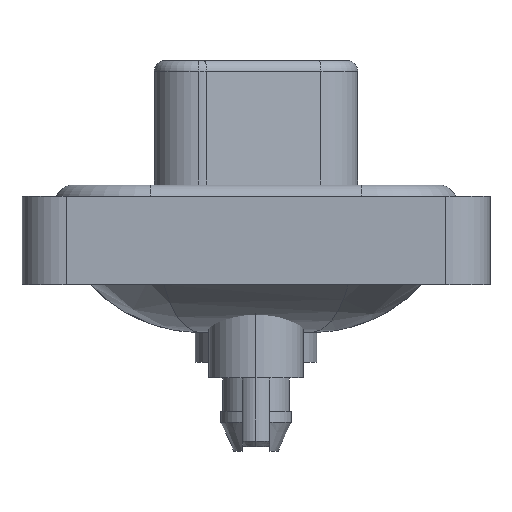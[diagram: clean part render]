
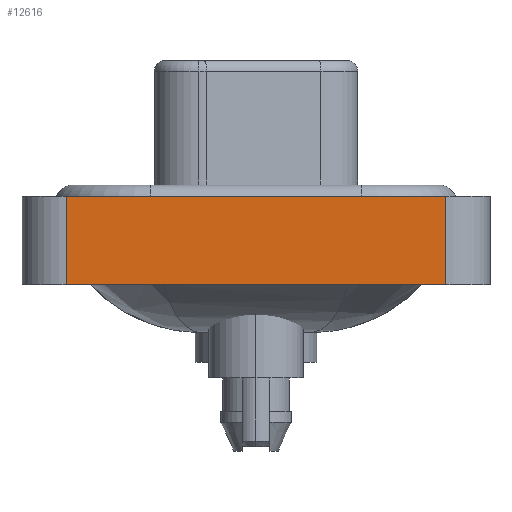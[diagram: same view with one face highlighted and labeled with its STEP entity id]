
A CAD part, left-side view. The second image highlights one B-rep face of the part: STEP entity #12616.
In plain terms, the highlighted planar face has unit normal (-1, 0, 0).
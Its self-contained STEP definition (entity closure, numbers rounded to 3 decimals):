
#95 = CARTESIAN_POINT ( 'NONE',  ( -7.25, 8.55, -3.6 ) ) ;
#122 = EDGE_CURVE ( 'NONE', #6247, #7674, #1466, .T. ) ;
#132 = LINE ( 'NONE', #12544, #2816 ) ;
#764 = CARTESIAN_POINT ( 'NONE',  ( -7.25, -8.55, 0.4 ) ) ;
#1466 = LINE ( 'NONE', #95, #2359 ) ;
#2124 = CARTESIAN_POINT ( 'NONE',  ( -7.25, 8.55, -3.6 ) ) ;
#2359 = VECTOR ( 'NONE', #2757, 1000. ) ;
#2703 = VECTOR ( 'NONE', #5706, 1000. ) ;
#2757 = DIRECTION ( 'NONE',  ( 0., 0., 1. ) ) ;
#2816 = VECTOR ( 'NONE', #13908, 1000. ) ;
#3711 = LINE ( 'NONE', #7516, #14394 ) ;
#4063 = CARTESIAN_POINT ( 'NONE',  ( -7.25, 8.55, 0.4 ) ) ;
#4376 = ORIENTED_EDGE ( 'NONE', *, *, #5754, .F. ) ;
#4644 = VERTEX_POINT ( 'NONE', #13628 ) ;
#5287 = ORIENTED_EDGE ( 'NONE', *, *, #11710, .T. ) ;
#5706 = DIRECTION ( 'NONE',  ( 0., -1., 0. ) ) ;
#5754 = EDGE_CURVE ( 'NONE', #7674, #15015, #9117, .T. ) ;
#5914 = AXIS2_PLACEMENT_3D ( 'NONE', #7771, #11454, #10336 ) ;
#6247 = VERTEX_POINT ( 'NONE', #2124 ) ;
#7322 = CARTESIAN_POINT ( 'NONE',  ( -7.25, -8.55, 0.4 ) ) ;
#7516 = CARTESIAN_POINT ( 'NONE',  ( -7.25, -8.55, -3.6 ) ) ;
#7674 = VERTEX_POINT ( 'NONE', #4063 ) ;
#7771 = CARTESIAN_POINT ( 'NONE',  ( -7.25, -8.55, -3.6 ) ) ;
#8980 = FACE_OUTER_BOUND ( 'NONE', #15879, .T. ) ;
#9117 = LINE ( 'NONE', #764, #2703 ) ;
#9148 = ORIENTED_EDGE ( 'NONE', *, *, #12907, .T. ) ;
#10336 = DIRECTION ( 'NONE',  ( 0., 0., 1. ) ) ;
#11454 = DIRECTION ( 'NONE',  ( -1., 0., 0. ) ) ;
#11710 = EDGE_CURVE ( 'NONE', #6247, #4644, #132, .T. ) ;
#12172 = DIRECTION ( 'NONE',  ( 0., 0., 1. ) ) ;
#12544 = CARTESIAN_POINT ( 'NONE',  ( -7.25, -8.55, -3.6 ) ) ;
#12616 = ADVANCED_FACE ( 'NONE', ( #8980 ), #13866, .T. ) ;
#12907 = EDGE_CURVE ( 'NONE', #4644, #15015, #3711, .T. ) ;
#13628 = CARTESIAN_POINT ( 'NONE',  ( -7.25, -8.55, -3.6 ) ) ;
#13866 = PLANE ( 'NONE',  #5914 ) ;
#13908 = DIRECTION ( 'NONE',  ( 0., -1., 0. ) ) ;
#14394 = VECTOR ( 'NONE', #12172, 1000. ) ;
#14444 = ORIENTED_EDGE ( 'NONE', *, *, #122, .F. ) ;
#15015 = VERTEX_POINT ( 'NONE', #7322 ) ;
#15879 = EDGE_LOOP ( 'NONE', ( #9148, #4376, #14444, #5287 ) ) ;
